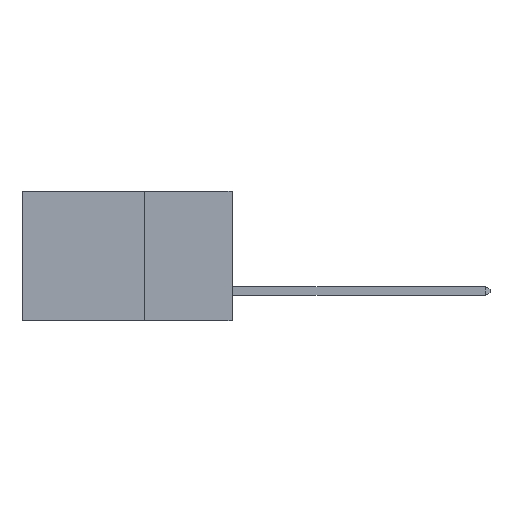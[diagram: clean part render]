
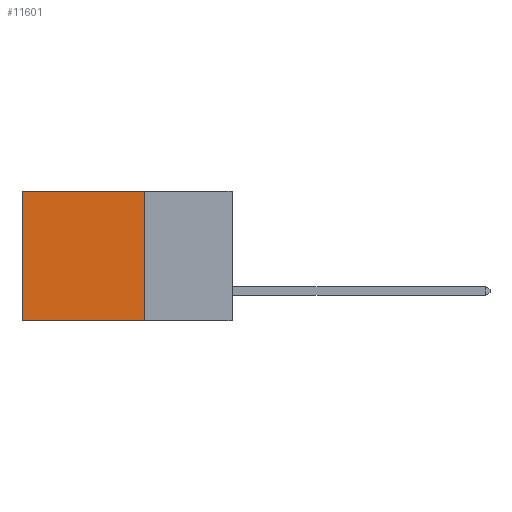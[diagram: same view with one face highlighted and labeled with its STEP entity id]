
A CAD part, left-side view. The second image highlights one B-rep face of the part: STEP entity #11601.
In plain terms, the highlighted planar face has unit normal (-1, 0, 0).
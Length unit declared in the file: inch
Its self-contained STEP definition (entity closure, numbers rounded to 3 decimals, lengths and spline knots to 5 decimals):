
#1673 = CARTESIAN_POINT ( 'NONE',  ( 0.2875, 0.25, 0. ) ) ;
#1788 = ORIENTED_EDGE ( 'NONE', *, *, #7930, .T. ) ;
#1810 = CARTESIAN_POINT ( 'NONE',  ( 0.2875, 0.6, 0. ) ) ;
#1952 = EDGE_LOOP ( 'NONE', ( #16569, #18006, #12496, #1788 ) ) ;
#3148 = LINE ( 'NONE', #18068, #24453 ) ;
#3270 = LINE ( 'NONE', #6560, #13697 ) ;
#3758 = DIRECTION ( 'NONE',  ( 0., 0., -1. ) ) ;
#5435 = FACE_OUTER_BOUND ( 'NONE', #1952, .T. ) ;
#6560 = CARTESIAN_POINT ( 'NONE',  ( 0.2875, 0.25, -0.37 ) ) ;
#7930 = EDGE_CURVE ( 'NONE', #17001, #8559, #17664, .T. ) ;
#8092 = VERTEX_POINT ( 'NONE', #18938 ) ;
#8559 = VERTEX_POINT ( 'NONE', #1810 ) ;
#8671 = DIRECTION ( 'NONE',  ( 0., 1., 0. ) ) ;
#11601 = ADVANCED_FACE ( 'NONE', ( #5435 ), #24223, .F. ) ;
#12247 = DIRECTION ( 'NONE',  ( 0., 1., 0. ) ) ;
#12496 = ORIENTED_EDGE ( 'NONE', *, *, #23659, .F. ) ;
#13148 = VERTEX_POINT ( 'NONE', #25134 ) ;
#13697 = VECTOR ( 'NONE', #8671, 39.37008 ) ;
#14522 = DIRECTION ( 'NONE',  ( 0., 0., -1. ) ) ;
#15082 = EDGE_CURVE ( 'NONE', #8092, #13148, #3270, .T. ) ;
#16220 = DIRECTION ( 'NONE',  ( 1., 0., 0. ) ) ;
#16540 = VECTOR ( 'NONE', #14522, 39.37008 ) ;
#16569 = ORIENTED_EDGE ( 'NONE', *, *, #17199, .T. ) ;
#17001 = VERTEX_POINT ( 'NONE', #19489 ) ;
#17034 = VECTOR ( 'NONE', #12247, 39.37008 ) ;
#17199 = EDGE_CURVE ( 'NONE', #8559, #13148, #3148, .T. ) ;
#17664 = LINE ( 'NONE', #20459, #17034 ) ;
#18006 = ORIENTED_EDGE ( 'NONE', *, *, #15082, .F. ) ;
#18068 = CARTESIAN_POINT ( 'NONE',  ( 0.2875, 0.6, 0. ) ) ;
#18938 = CARTESIAN_POINT ( 'NONE',  ( 0.2875, 0.25, -0.37 ) ) ;
#19489 = CARTESIAN_POINT ( 'NONE',  ( 0.2875, 0.25, 0. ) ) ;
#20114 = DIRECTION ( 'NONE',  ( 0., 0., -1. ) ) ;
#20459 = CARTESIAN_POINT ( 'NONE',  ( 0.2875, 0.25, 0. ) ) ;
#20491 = CARTESIAN_POINT ( 'NONE',  ( 0.2875, 0.25, 0. ) ) ;
#21453 = AXIS2_PLACEMENT_3D ( 'NONE', #1673, #16220, #3758 ) ;
#23235 = LINE ( 'NONE', #20491, #16540 ) ;
#23659 = EDGE_CURVE ( 'NONE', #17001, #8092, #23235, .T. ) ;
#24223 = PLANE ( 'NONE',  #21453 ) ;
#24453 = VECTOR ( 'NONE', #20114, 39.37008 ) ;
#25134 = CARTESIAN_POINT ( 'NONE',  ( 0.2875, 0.6, -0.37 ) ) ;
